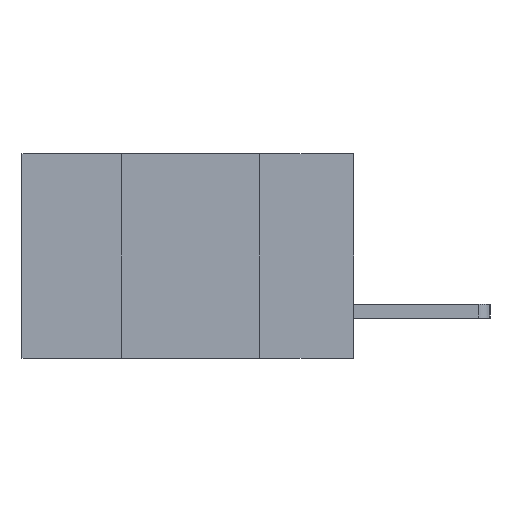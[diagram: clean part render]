
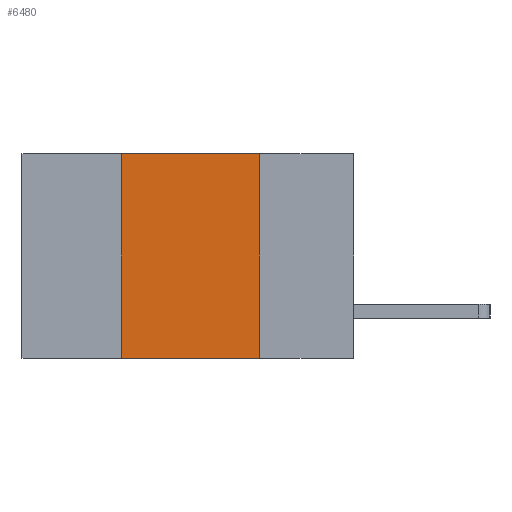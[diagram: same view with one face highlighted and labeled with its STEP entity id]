
A CAD part, left-side view. The second image highlights one B-rep face of the part: STEP entity #6480.
In plain terms, the highlighted planar face has unit normal (-1, 0, 0).
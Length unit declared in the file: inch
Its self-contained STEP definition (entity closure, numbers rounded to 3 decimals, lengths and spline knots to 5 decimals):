
#124 = EDGE_CURVE ( 'NONE', #5223, #9379, #4117, .T. ) ;
#160 = CARTESIAN_POINT ( 'NONE',  ( 0., 0.17, 0. ) ) ;
#168 = ORIENTED_EDGE ( 'NONE', *, *, #3618, .F. ) ;
#265 = LINE ( 'NONE', #160, #7154 ) ;
#551 = ORIENTED_EDGE ( 'NONE', *, *, #4971, .T. ) ;
#915 = DIRECTION ( 'NONE',  ( 0., 0., 1. ) ) ;
#1424 = DIRECTION ( 'NONE',  ( 0., 0., -1. ) ) ;
#1534 = DIRECTION ( 'NONE',  ( 0., -1., 0. ) ) ;
#1973 = AXIS2_PLACEMENT_3D ( 'NONE', #6143, #5378, #1424 ) ;
#2097 = VECTOR ( 'NONE', #915, 39.37008 ) ;
#2680 = VECTOR ( 'NONE', #9437, 39.37008 ) ;
#3618 = EDGE_CURVE ( 'NONE', #9379, #8451, #265, .T. ) ;
#3955 = EDGE_CURVE ( 'NONE', #5589, #5223, #6198, .T. ) ;
#3987 = CARTESIAN_POINT ( 'NONE',  ( 0., 0.17, 0. ) ) ;
#4014 = CARTESIAN_POINT ( 'NONE',  ( 0., 0.17, -0.37 ) ) ;
#4117 = LINE ( 'NONE', #6443, #2680 ) ;
#4478 = ORIENTED_EDGE ( 'NONE', *, *, #3955, .F. ) ;
#4611 = PLANE ( 'NONE',  #1973 ) ;
#4971 = EDGE_CURVE ( 'NONE', #5589, #8451, #7765, .T. ) ;
#5223 = VERTEX_POINT ( 'NONE', #8197 ) ;
#5378 = DIRECTION ( 'NONE',  ( 1., 0., 0. ) ) ;
#5542 = CARTESIAN_POINT ( 'NONE',  ( 0., 0.42, -0.37 ) ) ;
#5589 = VERTEX_POINT ( 'NONE', #5542 ) ;
#6038 = FACE_OUTER_BOUND ( 'NONE', #7967, .T. ) ;
#6143 = CARTESIAN_POINT ( 'NONE',  ( 0., 0.6, 0. ) ) ;
#6194 = VECTOR ( 'NONE', #1534, 39.37008 ) ;
#6198 = LINE ( 'NONE', #9296, #2097 ) ;
#6443 = CARTESIAN_POINT ( 'NONE',  ( 0., 0.6, 0. ) ) ;
#6480 = ADVANCED_FACE ( 'NONE', ( #6038 ), #4611, .F. ) ;
#7154 = VECTOR ( 'NONE', #8611, 39.37008 ) ;
#7568 = CARTESIAN_POINT ( 'NONE',  ( 0., 0.6, -0.37 ) ) ;
#7765 = LINE ( 'NONE', #7568, #6194 ) ;
#7967 = EDGE_LOOP ( 'NONE', ( #168, #8681, #4478, #551 ) ) ;
#8197 = CARTESIAN_POINT ( 'NONE',  ( 0., 0.42, 0. ) ) ;
#8451 = VERTEX_POINT ( 'NONE', #4014 ) ;
#8611 = DIRECTION ( 'NONE',  ( 0., 0., -1. ) ) ;
#8681 = ORIENTED_EDGE ( 'NONE', *, *, #124, .F. ) ;
#9296 = CARTESIAN_POINT ( 'NONE',  ( 0., 0.42, 0. ) ) ;
#9379 = VERTEX_POINT ( 'NONE', #3987 ) ;
#9437 = DIRECTION ( 'NONE',  ( 0., -1., 0. ) ) ;
